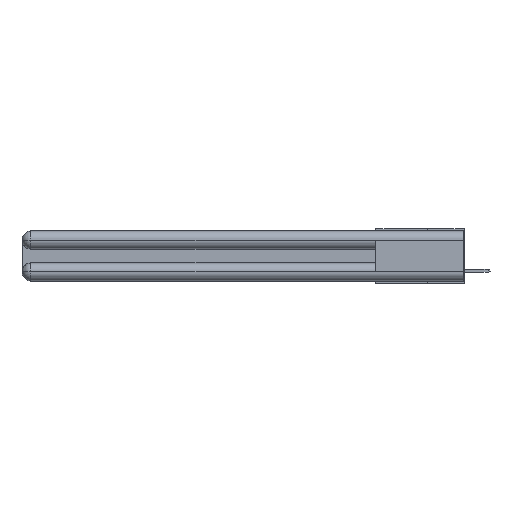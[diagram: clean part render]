
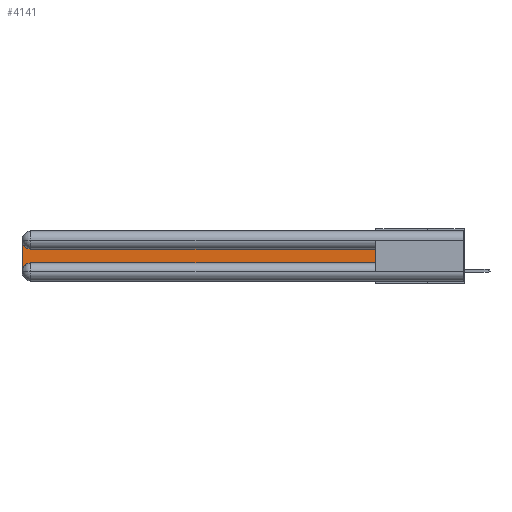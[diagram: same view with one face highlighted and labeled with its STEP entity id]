
A CAD part, left-side view. The second image highlights one B-rep face of the part: STEP entity #4141.
In plain terms, the highlighted planar face has unit normal (-1, 0, 0).
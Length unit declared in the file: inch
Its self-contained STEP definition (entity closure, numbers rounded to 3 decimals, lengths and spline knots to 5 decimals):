
#69 = VECTOR ( 'NONE', #10946, 39.37008 ) ;
#737 = CARTESIAN_POINT ( 'NONE',  ( 0.075, 0.6, -0.2175 ) ) ;
#929 = DIRECTION ( 'NONE',  ( 0., 0., -1. ) ) ;
#2280 = ORIENTED_EDGE ( 'NONE', *, *, #16838, .T. ) ;
#3354 = AXIS2_PLACEMENT_3D ( 'NONE', #5876, #20105, #18055 ) ;
#3557 = EDGE_CURVE ( 'NONE', #24552, #6681, #21339, .T. ) ;
#4132 = DIRECTION ( 'NONE',  ( 0., 0., -1. ) ) ;
#4141 = ADVANCED_FACE ( 'NONE', ( #14910 ), #15987, .F. ) ;
#4746 = CARTESIAN_POINT ( 'NONE',  ( 0.075, 2.94, -0.2175 ) ) ;
#5374 = VERTEX_POINT ( 'NONE', #16916 ) ;
#5401 = ORIENTED_EDGE ( 'NONE', *, *, #3557, .T. ) ;
#5545 = EDGE_LOOP ( 'NONE', ( #11191, #12697, #2280, #12504, #5401, #15299 ) ) ;
#5876 = CARTESIAN_POINT ( 'NONE',  ( 0.075, 3., -0.1225 ) ) ;
#6179 = CIRCLE ( 'NONE', #22608, 0.06 ) ;
#6681 = VERTEX_POINT ( 'NONE', #737 ) ;
#6769 = DIRECTION ( 'NONE',  ( 0., 0., 1. ) ) ;
#8827 = CARTESIAN_POINT ( 'NONE',  ( 0.075, 3., -0.0625 ) ) ;
#8980 = CARTESIAN_POINT ( 'NONE',  ( 0.075, 0.6, -0.1225 ) ) ;
#9102 = VERTEX_POINT ( 'NONE', #12559 ) ;
#9343 = LINE ( 'NONE', #14954, #25026 ) ;
#10946 = DIRECTION ( 'NONE',  ( 0., 1., 0. ) ) ;
#11191 = ORIENTED_EDGE ( 'NONE', *, *, #16017, .T. ) ;
#11212 = CARTESIAN_POINT ( 'NONE',  ( 0.075, 2.94, -0.0625 ) ) ;
#12504 = ORIENTED_EDGE ( 'NONE', *, *, #26455, .T. ) ;
#12559 = CARTESIAN_POINT ( 'NONE',  ( 0.075, 0.6, -0.1225 ) ) ;
#12697 = ORIENTED_EDGE ( 'NONE', *, *, #16323, .T. ) ;
#13120 = CARTESIAN_POINT ( 'NONE',  ( 0.075, 0.6, -0.2175 ) ) ;
#13250 = DIRECTION ( 'NONE',  ( 0., -1., 0. ) ) ;
#14329 = CARTESIAN_POINT ( 'NONE',  ( 0.075, 2.94, -0.2775 ) ) ;
#14910 = FACE_OUTER_BOUND ( 'NONE', #5545, .T. ) ;
#14954 = CARTESIAN_POINT ( 'NONE',  ( 0.075, 3., -0.2175 ) ) ;
#15299 = ORIENTED_EDGE ( 'NONE', *, *, #23935, .T. ) ;
#15383 = CARTESIAN_POINT ( 'NONE',  ( 0.075, 2.94, -0.1225 ) ) ;
#15987 = PLANE ( 'NONE',  #3354 ) ;
#16017 = EDGE_CURVE ( 'NONE', #9102, #16497, #26038, .T. ) ;
#16323 = EDGE_CURVE ( 'NONE', #16497, #22166, #6179, .T. ) ;
#16397 = DIRECTION ( 'NONE',  ( 1., 0., 0. ) ) ;
#16497 = VERTEX_POINT ( 'NONE', #15383 ) ;
#16838 = EDGE_CURVE ( 'NONE', #22166, #5374, #9343, .T. ) ;
#16916 = CARTESIAN_POINT ( 'NONE',  ( 0.075, 3., -0.2775 ) ) ;
#17270 = AXIS2_PLACEMENT_3D ( 'NONE', #14329, #16397, #4132 ) ;
#18055 = DIRECTION ( 'NONE',  ( 0., 0., -1. ) ) ;
#18805 = VECTOR ( 'NONE', #13250, 39.37008 ) ;
#18883 = VECTOR ( 'NONE', #6769, 39.37008 ) ;
#20105 = DIRECTION ( 'NONE',  ( 1., 0., 0. ) ) ;
#21339 = LINE ( 'NONE', #25501, #18805 ) ;
#22166 = VERTEX_POINT ( 'NONE', #8827 ) ;
#22608 = AXIS2_PLACEMENT_3D ( 'NONE', #11212, #25525, #929 ) ;
#23350 = DIRECTION ( 'NONE',  ( 0., 0., -1. ) ) ;
#23833 = CIRCLE ( 'NONE', #17270, 0.06 ) ;
#23935 = EDGE_CURVE ( 'NONE', #6681, #9102, #24310, .T. ) ;
#24310 = LINE ( 'NONE', #13120, #18883 ) ;
#24552 = VERTEX_POINT ( 'NONE', #4746 ) ;
#25026 = VECTOR ( 'NONE', #23350, 39.37008 ) ;
#25501 = CARTESIAN_POINT ( 'NONE',  ( 0.075, 0.6, -0.2175 ) ) ;
#25525 = DIRECTION ( 'NONE',  ( 1., 0., 0. ) ) ;
#26038 = LINE ( 'NONE', #8980, #69 ) ;
#26455 = EDGE_CURVE ( 'NONE', #5374, #24552, #23833, .T. ) ;
